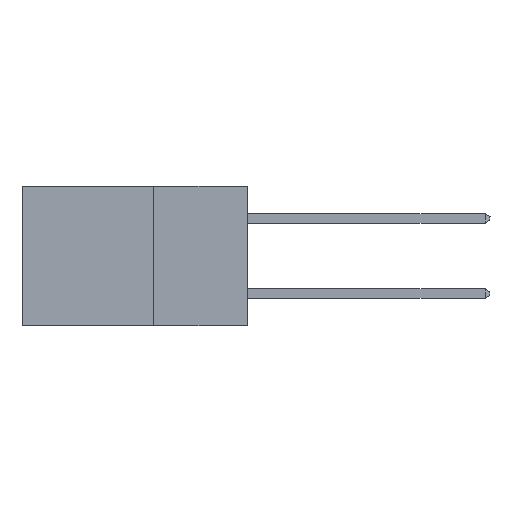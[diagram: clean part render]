
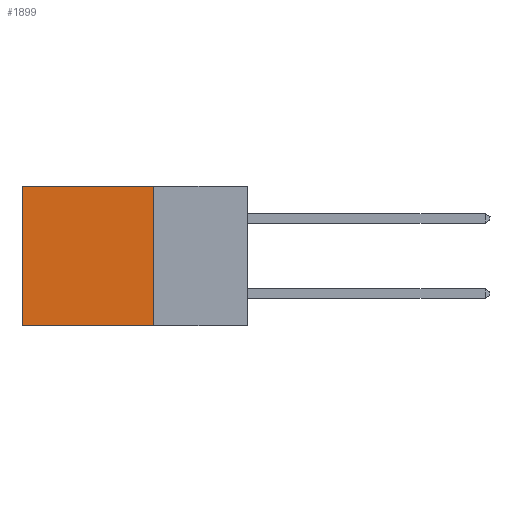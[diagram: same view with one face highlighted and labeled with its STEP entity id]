
A CAD part, left-side view. The second image highlights one B-rep face of the part: STEP entity #1899.
In plain terms, the highlighted planar face has unit normal (-1, 0, 0).
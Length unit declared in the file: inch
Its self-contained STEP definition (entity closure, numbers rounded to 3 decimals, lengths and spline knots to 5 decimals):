
#33 = LINE ( 'NONE', #10036, #17691 ) ;
#923 = VERTEX_POINT ( 'NONE', #11736 ) ;
#1433 = EDGE_CURVE ( 'NONE', #923, #5570, #33, .T. ) ;
#1899 = ADVANCED_FACE ( 'NONE', ( #7201 ), #11531, .F. ) ;
#2085 = LINE ( 'NONE', #13393, #13321 ) ;
#2734 = CARTESIAN_POINT ( 'NONE',  ( 0.2615, 0.25, -0.37 ) ) ;
#2922 = DIRECTION ( 'NONE',  ( 1., 0., 0. ) ) ;
#3098 = CARTESIAN_POINT ( 'NONE',  ( 0.2615, 0.25, -0.37 ) ) ;
#4189 = CARTESIAN_POINT ( 'NONE',  ( 0.2615, 0.6, -0.37 ) ) ;
#4202 = ORIENTED_EDGE ( 'NONE', *, *, #8181, .T. ) ;
#4449 = EDGE_CURVE ( 'NONE', #923, #5800, #2085, .T. ) ;
#5526 = EDGE_LOOP ( 'NONE', ( #4202, #16729, #9188, #11783 ) ) ;
#5570 = VERTEX_POINT ( 'NONE', #2734 ) ;
#5771 = VECTOR ( 'NONE', #13376, 39.37008 ) ;
#5800 = VERTEX_POINT ( 'NONE', #10112 ) ;
#7201 = FACE_OUTER_BOUND ( 'NONE', #5526, .T. ) ;
#7480 = AXIS2_PLACEMENT_3D ( 'NONE', #3098, #2922, #14609 ) ;
#7656 = EDGE_CURVE ( 'NONE', #5570, #10676, #9156, .T. ) ;
#8181 = EDGE_CURVE ( 'NONE', #5800, #10676, #16714, .T. ) ;
#8352 = DIRECTION ( 'NONE',  ( 0., 0., -1. ) ) ;
#9156 = LINE ( 'NONE', #13098, #5771 ) ;
#9188 = ORIENTED_EDGE ( 'NONE', *, *, #1433, .F. ) ;
#10036 = CARTESIAN_POINT ( 'NONE',  ( 0.2615, 0.25, -0.37 ) ) ;
#10112 = CARTESIAN_POINT ( 'NONE',  ( 0.2615, 0.6, 0. ) ) ;
#10676 = VERTEX_POINT ( 'NONE', #4189 ) ;
#11531 = PLANE ( 'NONE',  #7480 ) ;
#11555 = DIRECTION ( 'NONE',  ( 0., 0., -1. ) ) ;
#11736 = CARTESIAN_POINT ( 'NONE',  ( 0.2615, 0.25, 0. ) ) ;
#11783 = ORIENTED_EDGE ( 'NONE', *, *, #4449, .T. ) ;
#11794 = DIRECTION ( 'NONE',  ( 0., 1., 0. ) ) ;
#13098 = CARTESIAN_POINT ( 'NONE',  ( 0.2615, 0.25, -0.37 ) ) ;
#13321 = VECTOR ( 'NONE', #11794, 39.37008 ) ;
#13376 = DIRECTION ( 'NONE',  ( 0., 1., 0. ) ) ;
#13393 = CARTESIAN_POINT ( 'NONE',  ( 0.2615, 0.25, 0. ) ) ;
#14156 = CARTESIAN_POINT ( 'NONE',  ( 0.2615, 0.6, -0.37 ) ) ;
#14609 = DIRECTION ( 'NONE',  ( 0., 0., -1. ) ) ;
#16714 = LINE ( 'NONE', #14156, #18083 ) ;
#16729 = ORIENTED_EDGE ( 'NONE', *, *, #7656, .F. ) ;
#17691 = VECTOR ( 'NONE', #11555, 39.37008 ) ;
#18083 = VECTOR ( 'NONE', #8352, 39.37008 ) ;
